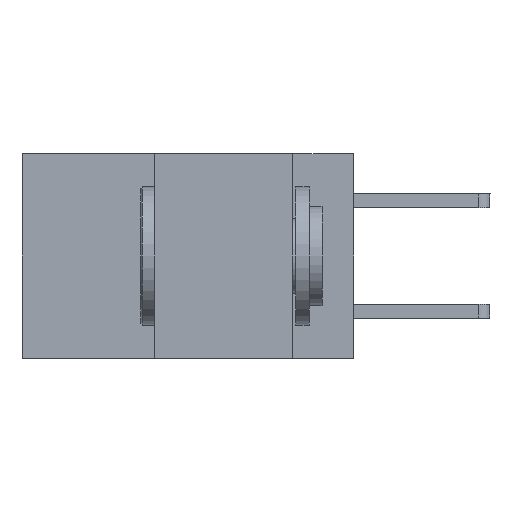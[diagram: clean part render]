
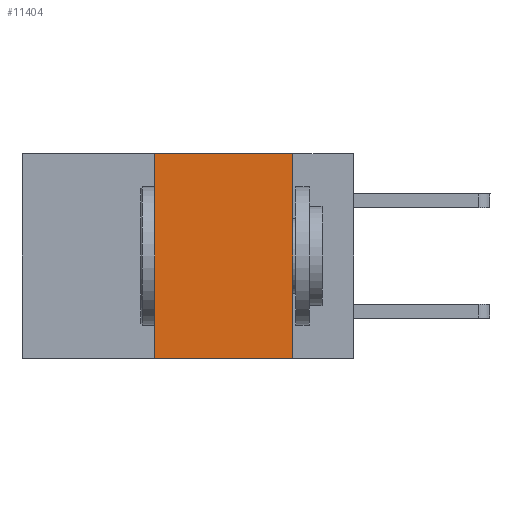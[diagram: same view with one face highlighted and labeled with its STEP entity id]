
A CAD part, left-side view. The second image highlights one B-rep face of the part: STEP entity #11404.
In plain terms, the highlighted planar face has unit normal (-1, 0, 0).
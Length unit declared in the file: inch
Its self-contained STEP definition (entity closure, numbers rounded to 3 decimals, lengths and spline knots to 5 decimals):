
#509 = DIRECTION ( 'NONE',  ( 1., 0., 0. ) ) ;
#725 = DIRECTION ( 'NONE',  ( 0., -1., 0. ) ) ;
#774 = AXIS2_PLACEMENT_3D ( 'NONE', #11239, #509, #10491 ) ;
#833 = FACE_OUTER_BOUND ( 'NONE', #10883, .T. ) ;
#968 = VERTEX_POINT ( 'NONE', #5927 ) ;
#1050 = VECTOR ( 'NONE', #725, 39.37008 ) ;
#1887 = LINE ( 'NONE', #4649, #11135 ) ;
#2008 = VERTEX_POINT ( 'NONE', #6628 ) ;
#2697 = VECTOR ( 'NONE', #3563, 39.37008 ) ;
#3045 = ORIENTED_EDGE ( 'NONE', *, *, #7543, .F. ) ;
#3108 = CARTESIAN_POINT ( 'NONE',  ( 0., 0.36, 0. ) ) ;
#3144 = PLANE ( 'NONE',  #774 ) ;
#3279 = ORIENTED_EDGE ( 'NONE', *, *, #8679, .T. ) ;
#3563 = DIRECTION ( 'NONE',  ( 0., 0., 1. ) ) ;
#3937 = VECTOR ( 'NONE', #7365, 39.37008 ) ;
#4031 = CARTESIAN_POINT ( 'NONE',  ( 0., 0.11, -0.37 ) ) ;
#4217 = LINE ( 'NONE', #6576, #3937 ) ;
#4266 = VERTEX_POINT ( 'NONE', #3108 ) ;
#4547 = ORIENTED_EDGE ( 'NONE', *, *, #5803, .F. ) ;
#4649 = CARTESIAN_POINT ( 'NONE',  ( 0., 0.11, 0. ) ) ;
#5749 = ORIENTED_EDGE ( 'NONE', *, *, #6646, .F. ) ;
#5803 = EDGE_CURVE ( 'NONE', #4266, #2008, #11154, .T. ) ;
#5927 = CARTESIAN_POINT ( 'NONE',  ( 0., 0.36, -0.37 ) ) ;
#6438 = DIRECTION ( 'NONE',  ( 0., 0., -1. ) ) ;
#6576 = CARTESIAN_POINT ( 'NONE',  ( 0., 0.6, -0.37 ) ) ;
#6628 = CARTESIAN_POINT ( 'NONE',  ( 0., 0.11, 0. ) ) ;
#6646 = EDGE_CURVE ( 'NONE', #2008, #9512, #1887, .T. ) ;
#7365 = DIRECTION ( 'NONE',  ( 0., -1., 0. ) ) ;
#7543 = EDGE_CURVE ( 'NONE', #968, #4266, #10717, .T. ) ;
#8679 = EDGE_CURVE ( 'NONE', #968, #9512, #4217, .T. ) ;
#8706 = CARTESIAN_POINT ( 'NONE',  ( 0., 0.6, 0. ) ) ;
#8958 = CARTESIAN_POINT ( 'NONE',  ( 0., 0.36, 0. ) ) ;
#9512 = VERTEX_POINT ( 'NONE', #4031 ) ;
#10491 = DIRECTION ( 'NONE',  ( 0., 0., -1. ) ) ;
#10717 = LINE ( 'NONE', #8958, #2697 ) ;
#10883 = EDGE_LOOP ( 'NONE', ( #5749, #4547, #3045, #3279 ) ) ;
#11135 = VECTOR ( 'NONE', #6438, 39.37008 ) ;
#11154 = LINE ( 'NONE', #8706, #1050 ) ;
#11239 = CARTESIAN_POINT ( 'NONE',  ( 0., 0.6, 0. ) ) ;
#11404 = ADVANCED_FACE ( 'NONE', ( #833 ), #3144, .F. ) ;
